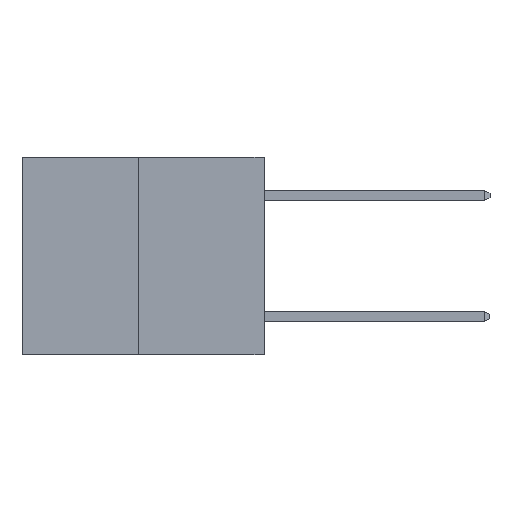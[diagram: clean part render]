
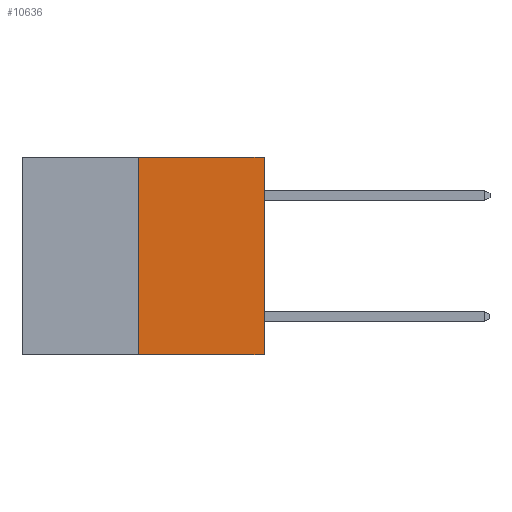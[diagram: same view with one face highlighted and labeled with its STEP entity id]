
A CAD part, left-side view. The second image highlights one B-rep face of the part: STEP entity #10636.
In plain terms, the highlighted planar face has unit normal (-1, 0, 0).
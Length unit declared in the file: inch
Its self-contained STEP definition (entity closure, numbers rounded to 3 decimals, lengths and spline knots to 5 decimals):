
#348 = EDGE_LOOP ( 'NONE', ( #16427, #15588, #13415, #19300 ) ) ;
#961 = EDGE_CURVE ( 'NONE', #11521, #15784, #2242, .T. ) ;
#1530 = DIRECTION ( 'NONE',  ( 0., 0., -1. ) ) ;
#1688 = LINE ( 'NONE', #6864, #18570 ) ;
#2008 = EDGE_CURVE ( 'NONE', #10123, #3907, #14975, .T. ) ;
#2242 = LINE ( 'NONE', #8652, #8512 ) ;
#3853 = FACE_OUTER_BOUND ( 'NONE', #348, .T. ) ;
#3907 = VERTEX_POINT ( 'NONE', #14512 ) ;
#4126 = VECTOR ( 'NONE', #14550, 39.37008 ) ;
#4568 = DIRECTION ( 'NONE',  ( 1., 0., 0. ) ) ;
#5640 = CARTESIAN_POINT ( 'NONE',  ( 0., 0., 0. ) ) ;
#6786 = VECTOR ( 'NONE', #12093, 39.37008 ) ;
#6793 = CARTESIAN_POINT ( 'NONE',  ( 0., 0.6, 0. ) ) ;
#6864 = CARTESIAN_POINT ( 'NONE',  ( 0., 0.6, -0.49 ) ) ;
#8512 = VECTOR ( 'NONE', #8585, 39.37008 ) ;
#8527 = AXIS2_PLACEMENT_3D ( 'NONE', #9223, #4568, #1530 ) ;
#8585 = DIRECTION ( 'NONE',  ( 0., 0., 1. ) ) ;
#8652 = CARTESIAN_POINT ( 'NONE',  ( 0., 0., 0. ) ) ;
#9223 = CARTESIAN_POINT ( 'NONE',  ( 0., 0.6, 0. ) ) ;
#10123 = VERTEX_POINT ( 'NONE', #12585 ) ;
#10636 = ADVANCED_FACE ( 'NONE', ( #3853 ), #12282, .F. ) ;
#10804 = EDGE_CURVE ( 'NONE', #10123, #11521, #1688, .T. ) ;
#11521 = VERTEX_POINT ( 'NONE', #17085 ) ;
#12093 = DIRECTION ( 'NONE',  ( 0., 0., 1. ) ) ;
#12160 = CARTESIAN_POINT ( 'NONE',  ( 0., 0.312, -0.49 ) ) ;
#12282 = PLANE ( 'NONE',  #8527 ) ;
#12352 = LINE ( 'NONE', #6793, #4126 ) ;
#12585 = CARTESIAN_POINT ( 'NONE',  ( 0., 0.312, -0.49 ) ) ;
#13415 = ORIENTED_EDGE ( 'NONE', *, *, #961, .T. ) ;
#14512 = CARTESIAN_POINT ( 'NONE',  ( 0., 0.312, 0. ) ) ;
#14550 = DIRECTION ( 'NONE',  ( 0., -1., 0. ) ) ;
#14975 = LINE ( 'NONE', #12160, #6786 ) ;
#15588 = ORIENTED_EDGE ( 'NONE', *, *, #10804, .T. ) ;
#15784 = VERTEX_POINT ( 'NONE', #5640 ) ;
#16427 = ORIENTED_EDGE ( 'NONE', *, *, #2008, .F. ) ;
#17085 = CARTESIAN_POINT ( 'NONE',  ( 0., 0., -0.49 ) ) ;
#17637 = EDGE_CURVE ( 'NONE', #3907, #15784, #12352, .T. ) ;
#18570 = VECTOR ( 'NONE', #19074, 39.37008 ) ;
#19074 = DIRECTION ( 'NONE',  ( 0., -1., 0. ) ) ;
#19300 = ORIENTED_EDGE ( 'NONE', *, *, #17637, .F. ) ;
